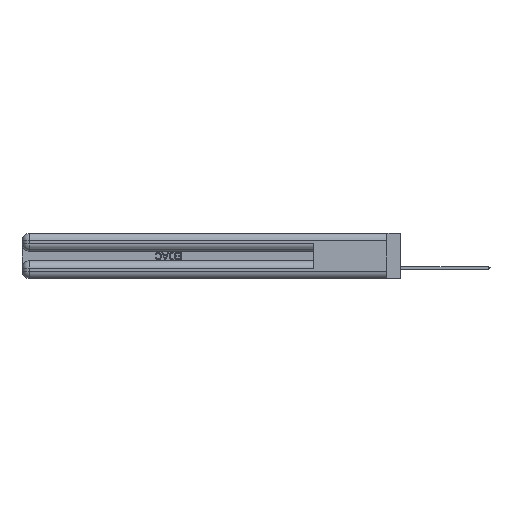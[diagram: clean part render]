
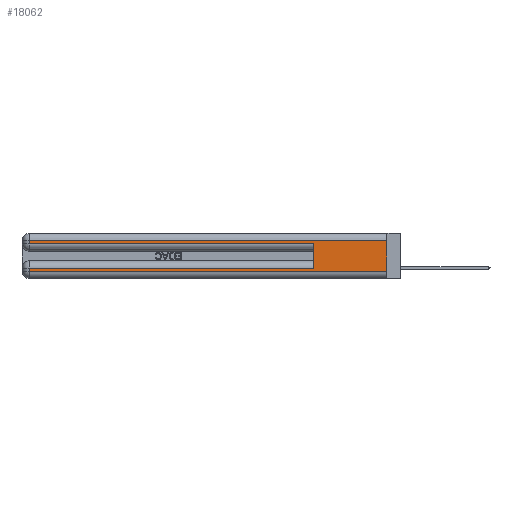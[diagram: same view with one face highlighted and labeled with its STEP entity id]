
A CAD part, left-side view. The second image highlights one B-rep face of the part: STEP entity #18062.
In plain terms, the highlighted planar face has unit normal (-1, 0, 0).
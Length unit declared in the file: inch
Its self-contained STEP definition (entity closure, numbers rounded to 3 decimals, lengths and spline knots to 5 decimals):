
#97 = ORIENTED_EDGE ( 'NONE', *, *, #1446, .T. ) ;
#1414 = CARTESIAN_POINT ( 'NONE',  ( 0., 0., 0.37 ) ) ;
#1446 = EDGE_CURVE ( 'NONE', #8624, #26096, #18796, .T. ) ;
#1990 = EDGE_CURVE ( 'NONE', #17081, #8624, #9332, .T. ) ;
#3264 = ORIENTED_EDGE ( 'NONE', *, *, #32855, .T. ) ;
#4689 = DIRECTION ( 'NONE',  ( 0., 0., -1. ) ) ;
#5232 = VECTOR ( 'NONE', #23887, 39.37008 ) ;
#5458 = LINE ( 'NONE', #32624, #29352 ) ;
#6443 = ORIENTED_EDGE ( 'NONE', *, *, #6767, .T. ) ;
#6719 = CARTESIAN_POINT ( 'NONE',  ( 0., 0., 0.085 ) ) ;
#6767 = EDGE_CURVE ( 'NONE', #16381, #17081, #37860, .T. ) ;
#6781 = VERTEX_POINT ( 'NONE', #41241 ) ;
#8294 = CARTESIAN_POINT ( 'NONE',  ( 0., 0., 0.06 ) ) ;
#8624 = VERTEX_POINT ( 'NONE', #36980 ) ;
#8829 = LINE ( 'NONE', #6719, #45543 ) ;
#9332 = LINE ( 'NONE', #22268, #37706 ) ;
#9402 = CARTESIAN_POINT ( 'NONE',  ( 0., 2.94, 0.31 ) ) ;
#9972 = VECTOR ( 'NONE', #23015, 39.37008 ) ;
#11017 = LINE ( 'NONE', #8294, #18781 ) ;
#11606 = CARTESIAN_POINT ( 'NONE',  ( 0., 0., 0.31 ) ) ;
#12204 = DIRECTION ( 'NONE',  ( 1., 0., 0. ) ) ;
#12228 = VECTOR ( 'NONE', #35077, 39.37008 ) ;
#14804 = AXIS2_PLACEMENT_3D ( 'NONE', #1414, #12204, #40628 ) ;
#15864 = DIRECTION ( 'NONE',  ( 0., 0., -1. ) ) ;
#16055 = DIRECTION ( 'NONE',  ( 0., -1., 0. ) ) ;
#16381 = VERTEX_POINT ( 'NONE', #11606 ) ;
#17081 = VERTEX_POINT ( 'NONE', #9402 ) ;
#17171 = CARTESIAN_POINT ( 'NONE',  ( 0., 0., 0.31 ) ) ;
#18062 = ADVANCED_FACE ( 'NONE', ( #18901 ), #44036, .F. ) ;
#18202 = VECTOR ( 'NONE', #15864, 39.37008 ) ;
#18240 = DIRECTION ( 'NONE',  ( 0., 0., -1. ) ) ;
#18781 = VECTOR ( 'NONE', #16055, 39.37008 ) ;
#18796 = LINE ( 'NONE', #19427, #9972 ) ;
#18901 = FACE_OUTER_BOUND ( 'NONE', #25569, .T. ) ;
#19427 = CARTESIAN_POINT ( 'NONE',  ( 0., 0., 0.285 ) ) ;
#19458 = EDGE_CURVE ( 'NONE', #6781, #36503, #8829, .T. ) ;
#20295 = CARTESIAN_POINT ( 'NONE',  ( 0., 0.6, 0.145 ) ) ;
#22268 = CARTESIAN_POINT ( 'NONE',  ( 0., 2.94, 0.37 ) ) ;
#23015 = DIRECTION ( 'NONE',  ( 0., -1., 0. ) ) ;
#23887 = DIRECTION ( 'NONE',  ( 0., 0., 1. ) ) ;
#24833 = ORIENTED_EDGE ( 'NONE', *, *, #33310, .F. ) ;
#25569 = EDGE_LOOP ( 'NONE', ( #24833, #6443, #27955, #97, #26028, #32182, #28279, #3264 ) ) ;
#26028 = ORIENTED_EDGE ( 'NONE', *, *, #29782, .F. ) ;
#26096 = VERTEX_POINT ( 'NONE', #40405 ) ;
#27955 = ORIENTED_EDGE ( 'NONE', *, *, #1990, .T. ) ;
#28279 = ORIENTED_EDGE ( 'NONE', *, *, #37445, .T. ) ;
#29352 = VECTOR ( 'NONE', #18240, 39.37008 ) ;
#29782 = EDGE_CURVE ( 'NONE', #6781, #26096, #30928, .T. ) ;
#30928 = LINE ( 'NONE', #20295, #5232 ) ;
#32182 = ORIENTED_EDGE ( 'NONE', *, *, #19458, .T. ) ;
#32624 = CARTESIAN_POINT ( 'NONE',  ( 0., 2.94, 0.37 ) ) ;
#32828 = VERTEX_POINT ( 'NONE', #36309 ) ;
#32855 = EDGE_CURVE ( 'NONE', #42942, #32828, #11017, .T. ) ;
#33310 = EDGE_CURVE ( 'NONE', #16381, #32828, #37130, .T. ) ;
#33688 = CARTESIAN_POINT ( 'NONE',  ( 0., 0., 0.37 ) ) ;
#35077 = DIRECTION ( 'NONE',  ( 0., 1., 0. ) ) ;
#36309 = CARTESIAN_POINT ( 'NONE',  ( 0., 0., 0.06 ) ) ;
#36503 = VERTEX_POINT ( 'NONE', #37324 ) ;
#36980 = CARTESIAN_POINT ( 'NONE',  ( 0., 2.94, 0.285 ) ) ;
#37130 = LINE ( 'NONE', #33688, #18202 ) ;
#37324 = CARTESIAN_POINT ( 'NONE',  ( 0., 2.94, 0.085 ) ) ;
#37445 = EDGE_CURVE ( 'NONE', #36503, #42942, #5458, .T. ) ;
#37706 = VECTOR ( 'NONE', #4689, 39.37008 ) ;
#37860 = LINE ( 'NONE', #17171, #12228 ) ;
#38461 = CARTESIAN_POINT ( 'NONE',  ( 0., 2.94, 0.06 ) ) ;
#40405 = CARTESIAN_POINT ( 'NONE',  ( 0., 0.6, 0.285 ) ) ;
#40628 = DIRECTION ( 'NONE',  ( 0., 0., -1. ) ) ;
#41241 = CARTESIAN_POINT ( 'NONE',  ( 0., 0.6, 0.085 ) ) ;
#42942 = VERTEX_POINT ( 'NONE', #38461 ) ;
#44036 = PLANE ( 'NONE',  #14804 ) ;
#45460 = DIRECTION ( 'NONE',  ( 0., 1., 0. ) ) ;
#45543 = VECTOR ( 'NONE', #45460, 39.37008 ) ;
